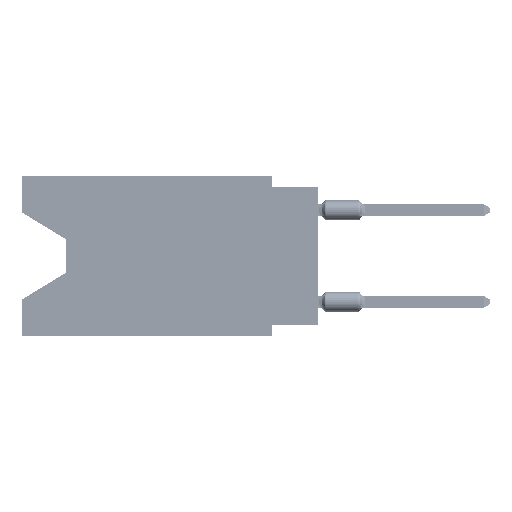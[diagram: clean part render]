
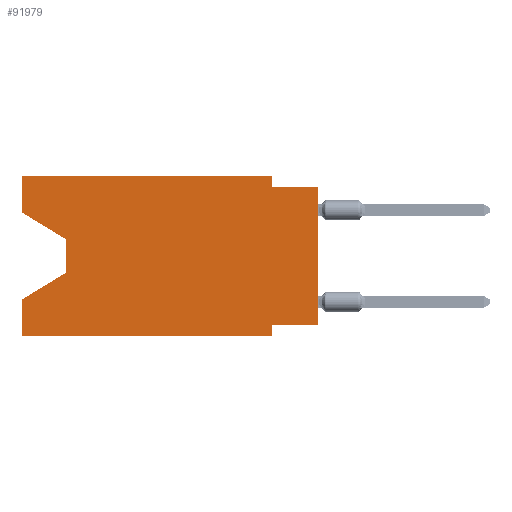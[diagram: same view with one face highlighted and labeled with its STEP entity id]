
A CAD part, left-side view. The second image highlights one B-rep face of the part: STEP entity #91979.
In plain terms, the highlighted planar face has unit normal (-1, 0, 0).
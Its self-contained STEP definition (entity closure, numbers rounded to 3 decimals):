
#958 = CARTESIAN_POINT ( 'NONE',  ( 0., 16.383, 0. ) ) ;
#1395 = CARTESIAN_POINT ( 'NONE',  ( 0., 0., -8.255 ) ) ;
#2293 = CARTESIAN_POINT ( 'NONE',  ( 0., 2.54, -8.255 ) ) ;
#3731 = VECTOR ( 'NONE', #18300, 1000. ) ;
#5170 = DIRECTION ( 'NONE',  ( 0., 0., -1. ) ) ;
#6794 = LINE ( 'NONE', #95808, #65284 ) ;
#6891 = ORIENTED_EDGE ( 'NONE', *, *, #81846, .F. ) ;
#7544 = ORIENTED_EDGE ( 'NONE', *, *, #54740, .F. ) ;
#7919 = VERTEX_POINT ( 'NONE', #63236 ) ;
#8227 = VECTOR ( 'NONE', #30159, 1000. ) ;
#8917 = DIRECTION ( 'NONE',  ( 1., 0., 0. ) ) ;
#9018 = VERTEX_POINT ( 'NONE', #33433 ) ;
#11385 = DIRECTION ( 'NONE',  ( 0., -1., 0. ) ) ;
#11416 = AXIS2_PLACEMENT_3D ( 'NONE', #958, #8917, #19308 ) ;
#14268 = VECTOR ( 'NONE', #11385, 1000. ) ;
#14874 = EDGE_CURVE ( 'NONE', #23390, #7919, #69684, .T. ) ;
#15424 = DIRECTION ( 'NONE',  ( 0., 0., -1. ) ) ;
#15783 = VERTEX_POINT ( 'NONE', #38008 ) ;
#16302 = DIRECTION ( 'NONE',  ( 0., 0., 1. ) ) ;
#17007 = CARTESIAN_POINT ( 'NONE',  ( 0., 0., -8.255 ) ) ;
#17174 = LINE ( 'NONE', #73331, #50519 ) ;
#18300 = DIRECTION ( 'NONE',  ( 0., 0.855, -0.519 ) ) ;
#19074 = VERTEX_POINT ( 'NONE', #31739 ) ;
#19308 = DIRECTION ( 'NONE',  ( 0., 0., -1. ) ) ;
#19700 = VERTEX_POINT ( 'NONE', #1395 ) ;
#20085 = DIRECTION ( 'NONE',  ( 0., 0., 1. ) ) ;
#21383 = VERTEX_POINT ( 'NONE', #95989 ) ;
#21588 = LINE ( 'NONE', #54424, #76970 ) ;
#22557 = ORIENTED_EDGE ( 'NONE', *, *, #27546, .F. ) ;
#23390 = VERTEX_POINT ( 'NONE', #102127 ) ;
#23671 = CARTESIAN_POINT ( 'NONE',  ( 0., 13.97, -3.505 ) ) ;
#26149 = ORIENTED_EDGE ( 'NONE', *, *, #54695, .T. ) ;
#27546 = EDGE_CURVE ( 'NONE', #15783, #52333, #17174, .T. ) ;
#29260 = ORIENTED_EDGE ( 'NONE', *, *, #103793, .T. ) ;
#29476 = EDGE_CURVE ( 'NONE', #19700, #68199, #48249, .T. ) ;
#29626 = CARTESIAN_POINT ( 'NONE',  ( 0., 16.383, -2.038 ) ) ;
#30159 = DIRECTION ( 'NONE',  ( 0., -0.855, -0.519 ) ) ;
#30325 = VERTEX_POINT ( 'NONE', #71341 ) ;
#31739 = CARTESIAN_POINT ( 'NONE',  ( 0., 16.383, 0. ) ) ;
#33093 = EDGE_CURVE ( 'NONE', #64137, #21383, #91920, .T. ) ;
#33433 = CARTESIAN_POINT ( 'NONE',  ( 0., 13.97, -3.505 ) ) ;
#34741 = VECTOR ( 'NONE', #15424, 1000. ) ;
#35118 = EDGE_LOOP ( 'NONE', ( #29260, #26149, #46805, #54582, #59864, #80686, #50545, #44636, #22557, #6891, #7544, #101548 ) ) ;
#38008 = CARTESIAN_POINT ( 'NONE',  ( 0., 2.54, -0.635 ) ) ;
#39265 = LINE ( 'NONE', #88049, #34741 ) ;
#42399 = LINE ( 'NONE', #74216, #63876 ) ;
#42890 = CARTESIAN_POINT ( 'NONE',  ( 0., 0., 0. ) ) ;
#44231 = CARTESIAN_POINT ( 'NONE',  ( 0., 16.383, -8.89 ) ) ;
#44636 = ORIENTED_EDGE ( 'NONE', *, *, #47515, .T. ) ;
#46347 = DIRECTION ( 'NONE',  ( 0., -1., 0. ) ) ;
#46398 = VECTOR ( 'NONE', #48016, 1000. ) ;
#46805 = ORIENTED_EDGE ( 'NONE', *, *, #33093, .T. ) ;
#47515 = EDGE_CURVE ( 'NONE', #19700, #52333, #91659, .T. ) ;
#48016 = DIRECTION ( 'NONE',  ( 0., 0., -1. ) ) ;
#48249 = LINE ( 'NONE', #17007, #76144 ) ;
#49581 = CARTESIAN_POINT ( 'NONE',  ( 0., 16.383, 0. ) ) ;
#50519 = VECTOR ( 'NONE', #81316, 1000. ) ;
#50545 = ORIENTED_EDGE ( 'NONE', *, *, #29476, .F. ) ;
#52333 = VERTEX_POINT ( 'NONE', #56983 ) ;
#54424 = CARTESIAN_POINT ( 'NONE',  ( 0., 2.54, -8.89 ) ) ;
#54582 = ORIENTED_EDGE ( 'NONE', *, *, #59371, .F. ) ;
#54695 = EDGE_CURVE ( 'NONE', #9018, #64137, #96273, .T. ) ;
#54740 = EDGE_CURVE ( 'NONE', #19074, #30325, #89895, .T. ) ;
#56983 = CARTESIAN_POINT ( 'NONE',  ( 0., 0., -0.635 ) ) ;
#59371 = EDGE_CURVE ( 'NONE', #23390, #21383, #42399, .T. ) ;
#59864 = ORIENTED_EDGE ( 'NONE', *, *, #14874, .T. ) ;
#63236 = CARTESIAN_POINT ( 'NONE',  ( 0., 2.54, -8.89 ) ) ;
#63876 = VECTOR ( 'NONE', #98091, 1000. ) ;
#64137 = VERTEX_POINT ( 'NONE', #82517 ) ;
#65233 = DIRECTION ( 'NONE',  ( 0., 1., 0. ) ) ;
#65284 = VECTOR ( 'NONE', #16302, 1000. ) ;
#67381 = VERTEX_POINT ( 'NONE', #78459 ) ;
#68199 = VERTEX_POINT ( 'NONE', #2293 ) ;
#69684 = LINE ( 'NONE', #44231, #96675 ) ;
#70447 = LINE ( 'NONE', #29626, #8227 ) ;
#71341 = CARTESIAN_POINT ( 'NONE',  ( 0., 2.54, 0. ) ) ;
#73331 = CARTESIAN_POINT ( 'NONE',  ( 0., 0., -0.635 ) ) ;
#73543 = PLANE ( 'NONE',  #11416 ) ;
#74216 = CARTESIAN_POINT ( 'NONE',  ( 0., 16.383, 0. ) ) ;
#75554 = VECTOR ( 'NONE', #20085, 1000. ) ;
#76008 = FACE_OUTER_BOUND ( 'NONE', #35118, .T. ) ;
#76144 = VECTOR ( 'NONE', #65233, 1000. ) ;
#76970 = VECTOR ( 'NONE', #5170, 1000. ) ;
#78459 = CARTESIAN_POINT ( 'NONE',  ( 0., 16.383, -2.038 ) ) ;
#80686 = ORIENTED_EDGE ( 'NONE', *, *, #97781, .F. ) ;
#81316 = DIRECTION ( 'NONE',  ( 0., -1., 0. ) ) ;
#81846 = EDGE_CURVE ( 'NONE', #30325, #15783, #39265, .T. ) ;
#82517 = CARTESIAN_POINT ( 'NONE',  ( 0., 13.97, -5.385 ) ) ;
#88049 = CARTESIAN_POINT ( 'NONE',  ( 0., 2.54, 0. ) ) ;
#89895 = LINE ( 'NONE', #49581, #14268 ) ;
#91659 = LINE ( 'NONE', #42890, #75554 ) ;
#91920 = LINE ( 'NONE', #98845, #3731 ) ;
#91979 = ADVANCED_FACE ( 'NONE', ( #76008 ), #73543, .F. ) ;
#95808 = CARTESIAN_POINT ( 'NONE',  ( 0., 16.383, 0. ) ) ;
#95989 = CARTESIAN_POINT ( 'NONE',  ( 0., 16.383, -6.852 ) ) ;
#96273 = LINE ( 'NONE', #23671, #46398 ) ;
#96675 = VECTOR ( 'NONE', #46347, 1000. ) ;
#97781 = EDGE_CURVE ( 'NONE', #68199, #7919, #21588, .T. ) ;
#98091 = DIRECTION ( 'NONE',  ( 0., 0., 1. ) ) ;
#98733 = EDGE_CURVE ( 'NONE', #67381, #19074, #6794, .T. ) ;
#98845 = CARTESIAN_POINT ( 'NONE',  ( 0., 13.97, -5.385 ) ) ;
#101548 = ORIENTED_EDGE ( 'NONE', *, *, #98733, .F. ) ;
#102127 = CARTESIAN_POINT ( 'NONE',  ( 0., 16.383, -8.89 ) ) ;
#103793 = EDGE_CURVE ( 'NONE', #67381, #9018, #70447, .T. ) ;
